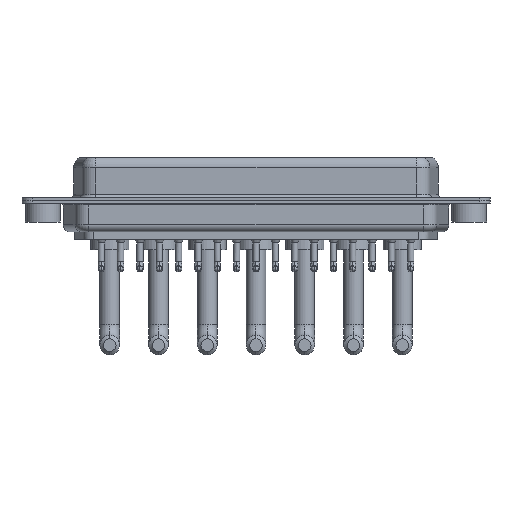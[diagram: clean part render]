
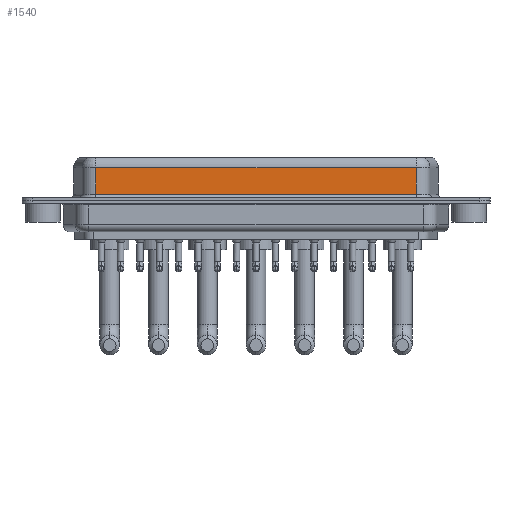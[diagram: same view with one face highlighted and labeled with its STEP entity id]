
A CAD part, front view. The second image highlights one B-rep face of the part: STEP entity #1540.
In plain terms, the highlighted planar face has unit normal (0, -1, 0).
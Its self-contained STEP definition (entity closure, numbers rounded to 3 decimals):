
#1540 = ADVANCED_FACE ( 'NONE', ( #13645 ), #14189, .F. ) ;
#1714 = VERTEX_POINT ( 'NONE', #21128 ) ;
#2622 = ORIENTED_EDGE ( 'NONE', *, *, #3416, .F. ) ;
#3416 = EDGE_CURVE ( 'NONE', #13044, #13520, #19697, .T. ) ;
#4008 = EDGE_LOOP ( 'NONE', ( #2622, #15020, #16974, #4894 ) ) ;
#4894 = ORIENTED_EDGE ( 'NONE', *, *, #16086, .T. ) ;
#4911 = CARTESIAN_POINT ( 'NONE',  ( 53.41, -5.375, 0.9 ) ) ;
#5920 = CARTESIAN_POINT ( 'NONE',  ( 53.41, -5.375, 4.65 ) ) ;
#6706 = VECTOR ( 'NONE', #13585, 1000. ) ;
#6733 = CARTESIAN_POINT ( 'NONE',  ( 53.41, -5.375, 6.4 ) ) ;
#7896 = CARTESIAN_POINT ( 'NONE',  ( 7.59, -5.375, 4.65 ) ) ;
#9045 = DIRECTION ( 'NONE',  ( 0., 1., 0. ) ) ;
#9090 = LINE ( 'NONE', #12191, #6706 ) ;
#9345 = VECTOR ( 'NONE', #11351, 1000. ) ;
#9650 = VECTOR ( 'NONE', #19301, 1000. ) ;
#10858 = CARTESIAN_POINT ( 'NONE',  ( 53.41, -5.375, 6.4 ) ) ;
#10954 = CARTESIAN_POINT ( 'NONE',  ( 7.59, -5.375, 6.4 ) ) ;
#11351 = DIRECTION ( 'NONE',  ( 1., 0., 0. ) ) ;
#12191 = CARTESIAN_POINT ( 'NONE',  ( 53.41, -5.375, 4.65 ) ) ;
#12733 = AXIS2_PLACEMENT_3D ( 'NONE', #10858, #9045, #20707 ) ;
#13044 = VERTEX_POINT ( 'NONE', #5920 ) ;
#13045 = CARTESIAN_POINT ( 'NONE',  ( 53.41, -5.375, 0.9 ) ) ;
#13370 = DIRECTION ( 'NONE',  ( 0., 0., -1. ) ) ;
#13520 = VERTEX_POINT ( 'NONE', #13045 ) ;
#13585 = DIRECTION ( 'NONE',  ( -1., 0., 0. ) ) ;
#13645 = FACE_OUTER_BOUND ( 'NONE', #4008, .T. ) ;
#14189 = PLANE ( 'NONE',  #12733 ) ;
#15020 = ORIENTED_EDGE ( 'NONE', *, *, #17617, .T. ) ;
#16086 = EDGE_CURVE ( 'NONE', #1714, #13520, #16466, .T. ) ;
#16466 = LINE ( 'NONE', #4911, #9345 ) ;
#16974 = ORIENTED_EDGE ( 'NONE', *, *, #21089, .T. ) ;
#17617 = EDGE_CURVE ( 'NONE', #13044, #20192, #9090, .T. ) ;
#19301 = DIRECTION ( 'NONE',  ( 0., 0., -1. ) ) ;
#19619 = VECTOR ( 'NONE', #13370, 1000. ) ;
#19697 = LINE ( 'NONE', #6733, #19619 ) ;
#20192 = VERTEX_POINT ( 'NONE', #7896 ) ;
#20584 = LINE ( 'NONE', #10954, #9650 ) ;
#20707 = DIRECTION ( 'NONE',  ( 0., 0., 1. ) ) ;
#21089 = EDGE_CURVE ( 'NONE', #20192, #1714, #20584, .T. ) ;
#21128 = CARTESIAN_POINT ( 'NONE',  ( 7.59, -5.375, 0.9 ) ) ;
